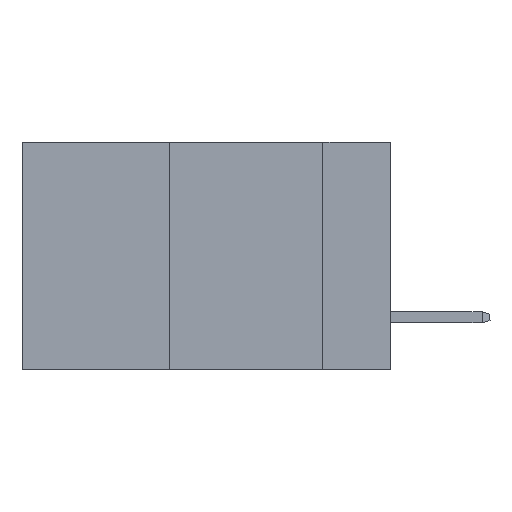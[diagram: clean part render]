
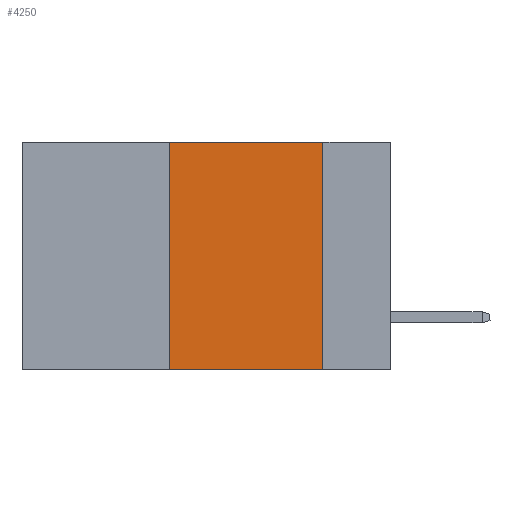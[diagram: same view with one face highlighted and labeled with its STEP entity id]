
A CAD part, left-side view. The second image highlights one B-rep face of the part: STEP entity #4250.
In plain terms, the highlighted planar face has unit normal (-1, 0, 0).
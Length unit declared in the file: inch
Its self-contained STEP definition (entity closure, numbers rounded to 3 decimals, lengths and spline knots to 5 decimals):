
#7 = CARTESIAN_POINT ( 'NONE',  ( 0., 0.36, -0.37 ) ) ;
#89 = VERTEX_POINT ( 'NONE', #13832 ) ;
#185 = CARTESIAN_POINT ( 'NONE',  ( 0., 0.36, 0. ) ) ;
#1012 = DIRECTION ( 'NONE',  ( 0., 0., 1. ) ) ;
#1081 = EDGE_CURVE ( 'NONE', #13329, #89, #3319, .T. ) ;
#1097 = VERTEX_POINT ( 'NONE', #7 ) ;
#1643 = ORIENTED_EDGE ( 'NONE', *, *, #6054, .T. ) ;
#2409 = PLANE ( 'NONE',  #13082 ) ;
#2413 = LINE ( 'NONE', #3611, #11168 ) ;
#2543 = LINE ( 'NONE', #3517, #3056 ) ;
#3056 = VECTOR ( 'NONE', #4516, 39.37008 ) ;
#3319 = LINE ( 'NONE', #11163, #12777 ) ;
#3517 = CARTESIAN_POINT ( 'NONE',  ( 0., 0.6, -0.37 ) ) ;
#3611 = CARTESIAN_POINT ( 'NONE',  ( 0., 0.36, 0. ) ) ;
#3710 = EDGE_LOOP ( 'NONE', ( #8986, #7966, #13684, #1643 ) ) ;
#4250 = ADVANCED_FACE ( 'NONE', ( #11876 ), #2409, .F. ) ;
#4516 = DIRECTION ( 'NONE',  ( 0., -1., 0. ) ) ;
#4646 = EDGE_CURVE ( 'NONE', #1097, #9331, #2413, .T. ) ;
#5709 = CARTESIAN_POINT ( 'NONE',  ( 0., 0.11, 0. ) ) ;
#6054 = EDGE_CURVE ( 'NONE', #1097, #89, #2543, .T. ) ;
#6846 = DIRECTION ( 'NONE',  ( 0., 0., -1. ) ) ;
#6847 = DIRECTION ( 'NONE',  ( 1., 0., 0. ) ) ;
#7705 = CARTESIAN_POINT ( 'NONE',  ( 0., 0.6, 0. ) ) ;
#7763 = EDGE_CURVE ( 'NONE', #9331, #13329, #10065, .T. ) ;
#7966 = ORIENTED_EDGE ( 'NONE', *, *, #7763, .F. ) ;
#8986 = ORIENTED_EDGE ( 'NONE', *, *, #1081, .F. ) ;
#9009 = DIRECTION ( 'NONE',  ( 0., 0., -1. ) ) ;
#9331 = VERTEX_POINT ( 'NONE', #185 ) ;
#9564 = VECTOR ( 'NONE', #12190, 39.37008 ) ;
#10065 = LINE ( 'NONE', #7705, #9564 ) ;
#11163 = CARTESIAN_POINT ( 'NONE',  ( 0., 0.11, 0. ) ) ;
#11168 = VECTOR ( 'NONE', #1012, 39.37008 ) ;
#11876 = FACE_OUTER_BOUND ( 'NONE', #3710, .T. ) ;
#12190 = DIRECTION ( 'NONE',  ( 0., -1., 0. ) ) ;
#12777 = VECTOR ( 'NONE', #6846, 39.37008 ) ;
#13082 = AXIS2_PLACEMENT_3D ( 'NONE', #13417, #6847, #9009 ) ;
#13329 = VERTEX_POINT ( 'NONE', #5709 ) ;
#13417 = CARTESIAN_POINT ( 'NONE',  ( 0., 0.6, 0. ) ) ;
#13684 = ORIENTED_EDGE ( 'NONE', *, *, #4646, .F. ) ;
#13832 = CARTESIAN_POINT ( 'NONE',  ( 0., 0.11, -0.37 ) ) ;
